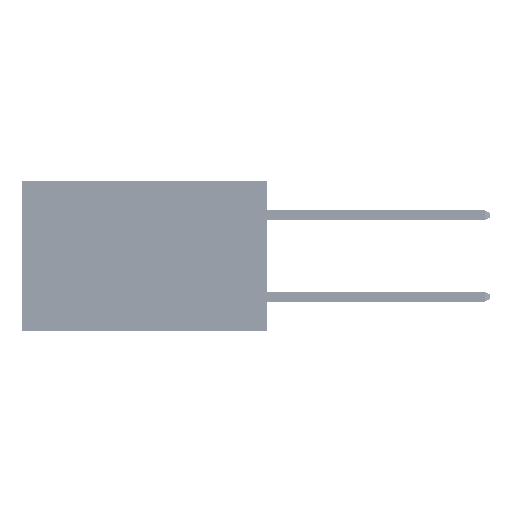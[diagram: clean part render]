
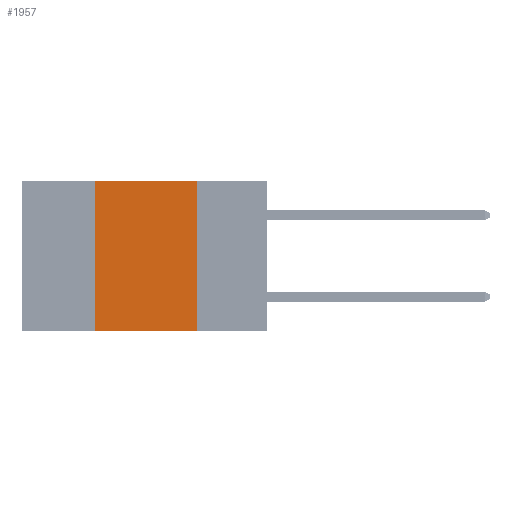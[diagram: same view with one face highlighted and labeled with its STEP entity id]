
A CAD part, left-side view. The second image highlights one B-rep face of the part: STEP entity #1957.
In plain terms, the highlighted planar face has unit normal (-1, 0, 0).
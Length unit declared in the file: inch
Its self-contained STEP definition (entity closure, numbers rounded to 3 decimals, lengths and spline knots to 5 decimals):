
#209 = EDGE_CURVE ( 'NONE', #12447, #39344, #4972, .T. ) ;
#1311 = ORIENTED_EDGE ( 'NONE', *, *, #26517, .F. ) ;
#1878 = CARTESIAN_POINT ( 'NONE',  ( 0., 0.6, -0.37 ) ) ;
#1957 = ADVANCED_FACE ( 'NONE', ( #26584 ), #20879, .F. ) ;
#3470 = LINE ( 'NONE', #42251, #40305 ) ;
#3563 = CARTESIAN_POINT ( 'NONE',  ( 0., 0.42, 0. ) ) ;
#4972 = LINE ( 'NONE', #26366, #30350 ) ;
#8005 = ORIENTED_EDGE ( 'NONE', *, *, #8420, .T. ) ;
#8420 = EDGE_CURVE ( 'NONE', #27473, #39344, #12468, .T. ) ;
#9259 = DIRECTION ( 'NONE',  ( 1., 0., 0. ) ) ;
#10331 = DIRECTION ( 'NONE',  ( 0., -1., 0. ) ) ;
#12447 = VERTEX_POINT ( 'NONE', #19388 ) ;
#12468 = LINE ( 'NONE', #1878, #31764 ) ;
#15148 = EDGE_LOOP ( 'NONE', ( #46459, #1311, #40435, #8005 ) ) ;
#16115 = EDGE_CURVE ( 'NONE', #27473, #27232, #3470, .T. ) ;
#16480 = DIRECTION ( 'NONE',  ( 0., 0., -1. ) ) ;
#16886 = AXIS2_PLACEMENT_3D ( 'NONE', #47785, #9259, #16480 ) ;
#19388 = CARTESIAN_POINT ( 'NONE',  ( 0., 0.17, 0. ) ) ;
#20879 = PLANE ( 'NONE',  #16886 ) ;
#21455 = DIRECTION ( 'NONE',  ( 0., -1., 0. ) ) ;
#24687 = LINE ( 'NONE', #33418, #40361 ) ;
#26366 = CARTESIAN_POINT ( 'NONE',  ( 0., 0.17, 0. ) ) ;
#26517 = EDGE_CURVE ( 'NONE', #27232, #12447, #24687, .T. ) ;
#26584 = FACE_OUTER_BOUND ( 'NONE', #15148, .T. ) ;
#26896 = DIRECTION ( 'NONE',  ( 0., 0., 1. ) ) ;
#27232 = VERTEX_POINT ( 'NONE', #3563 ) ;
#27473 = VERTEX_POINT ( 'NONE', #35611 ) ;
#30350 = VECTOR ( 'NONE', #30424, 39.37008 ) ;
#30424 = DIRECTION ( 'NONE',  ( 0., 0., -1. ) ) ;
#31764 = VECTOR ( 'NONE', #21455, 39.37008 ) ;
#33275 = CARTESIAN_POINT ( 'NONE',  ( 0., 0.17, -0.37 ) ) ;
#33418 = CARTESIAN_POINT ( 'NONE',  ( 0., 0.6, 0. ) ) ;
#35611 = CARTESIAN_POINT ( 'NONE',  ( 0., 0.42, -0.37 ) ) ;
#39344 = VERTEX_POINT ( 'NONE', #33275 ) ;
#40305 = VECTOR ( 'NONE', #26896, 39.37008 ) ;
#40361 = VECTOR ( 'NONE', #10331, 39.37008 ) ;
#40435 = ORIENTED_EDGE ( 'NONE', *, *, #16115, .F. ) ;
#42251 = CARTESIAN_POINT ( 'NONE',  ( 0., 0.42, 0. ) ) ;
#46459 = ORIENTED_EDGE ( 'NONE', *, *, #209, .F. ) ;
#47785 = CARTESIAN_POINT ( 'NONE',  ( 0., 0.6, 0. ) ) ;
